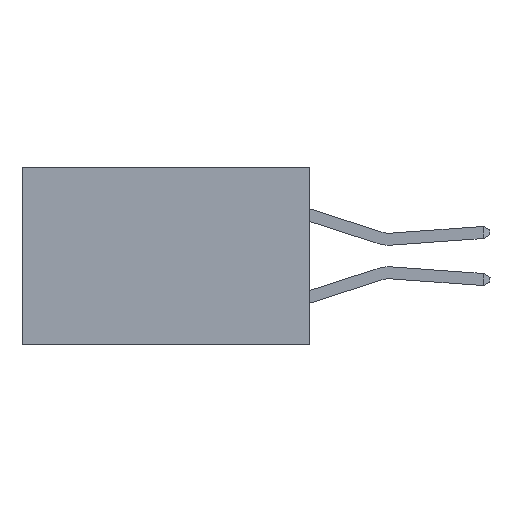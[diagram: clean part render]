
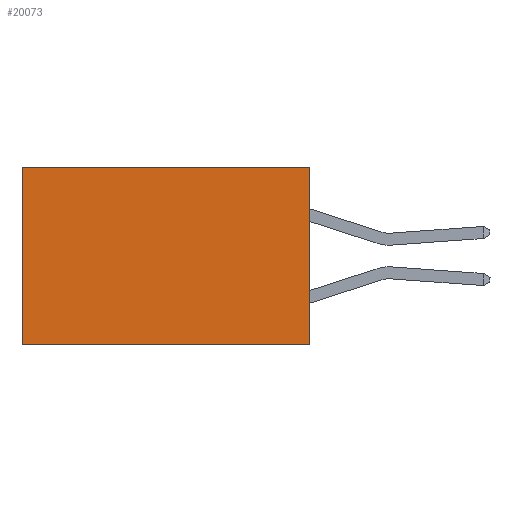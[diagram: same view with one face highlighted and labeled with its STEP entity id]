
A CAD part, left-side view. The second image highlights one B-rep face of the part: STEP entity #20073.
In plain terms, the highlighted planar face has unit normal (-1, 0, 0).
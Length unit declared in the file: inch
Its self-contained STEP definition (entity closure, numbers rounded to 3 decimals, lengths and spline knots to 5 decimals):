
#371 = DIRECTION ( 'NONE',  ( 0., 0., -1. ) ) ;
#1367 = EDGE_CURVE ( 'NONE', #15101, #3859, #29661, .T. ) ;
#2230 = DIRECTION ( 'NONE',  ( 0., 1., 0. ) ) ;
#3047 = VECTOR ( 'NONE', #17366, 39.37008 ) ;
#3859 = VERTEX_POINT ( 'NONE', #16875 ) ;
#4186 = CARTESIAN_POINT ( 'NONE',  ( 0.298, 0.6, 0. ) ) ;
#4206 = DIRECTION ( 'NONE',  ( 0., 0., -1. ) ) ;
#4526 = CARTESIAN_POINT ( 'NONE',  ( 0.298, 0.6, 0. ) ) ;
#6076 = FACE_OUTER_BOUND ( 'NONE', #23826, .T. ) ;
#6284 = VECTOR ( 'NONE', #371, 39.37008 ) ;
#7557 = CARTESIAN_POINT ( 'NONE',  ( 0.298, 0., 0. ) ) ;
#8773 = ORIENTED_EDGE ( 'NONE', *, *, #25957, .F. ) ;
#9777 = CARTESIAN_POINT ( 'NONE',  ( 0.298, 0., -0.37 ) ) ;
#10558 = ORIENTED_EDGE ( 'NONE', *, *, #16811, .T. ) ;
#13335 = ORIENTED_EDGE ( 'NONE', *, *, #20168, .T. ) ;
#14096 = LINE ( 'NONE', #22902, #6284 ) ;
#14264 = PLANE ( 'NONE',  #26268 ) ;
#14793 = VERTEX_POINT ( 'NONE', #7557 ) ;
#15101 = VERTEX_POINT ( 'NONE', #9777 ) ;
#15446 = VECTOR ( 'NONE', #2230, 39.37008 ) ;
#15447 = VECTOR ( 'NONE', #27068, 39.37008 ) ;
#16226 = LINE ( 'NONE', #24425, #15446 ) ;
#16811 = EDGE_CURVE ( 'NONE', #20850, #3859, #31870, .T. ) ;
#16875 = CARTESIAN_POINT ( 'NONE',  ( 0.298, 0.6, -0.37 ) ) ;
#17366 = DIRECTION ( 'NONE',  ( 0., 1., 0. ) ) ;
#19192 = DIRECTION ( 'NONE',  ( 1., 0., 0. ) ) ;
#20073 = ADVANCED_FACE ( 'NONE', ( #6076 ), #14264, .F. ) ;
#20168 = EDGE_CURVE ( 'NONE', #14793, #20850, #16226, .T. ) ;
#20850 = VERTEX_POINT ( 'NONE', #4186 ) ;
#22902 = CARTESIAN_POINT ( 'NONE',  ( 0.298, 0., 0. ) ) ;
#23826 = EDGE_LOOP ( 'NONE', ( #10558, #29074, #8773, #13335 ) ) ;
#24425 = CARTESIAN_POINT ( 'NONE',  ( 0.298, 0., 0. ) ) ;
#25957 = EDGE_CURVE ( 'NONE', #14793, #15101, #14096, .T. ) ;
#26268 = AXIS2_PLACEMENT_3D ( 'NONE', #31541, #19192, #4206 ) ;
#27068 = DIRECTION ( 'NONE',  ( 0., 0., -1. ) ) ;
#29074 = ORIENTED_EDGE ( 'NONE', *, *, #1367, .F. ) ;
#29661 = LINE ( 'NONE', #32251, #3047 ) ;
#31541 = CARTESIAN_POINT ( 'NONE',  ( 0.298, 0., 0. ) ) ;
#31870 = LINE ( 'NONE', #4526, #15447 ) ;
#32251 = CARTESIAN_POINT ( 'NONE',  ( 0.298, 0., -0.37 ) ) ;
